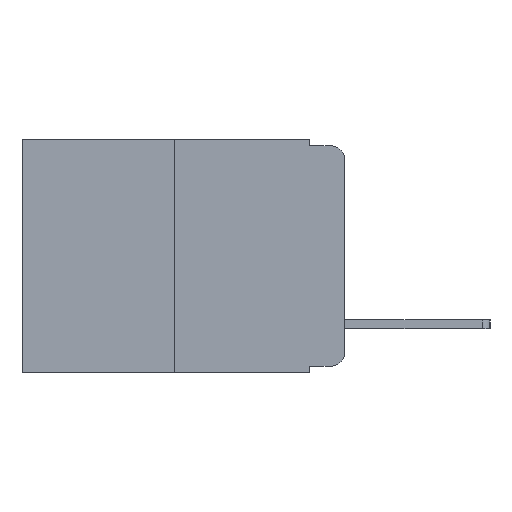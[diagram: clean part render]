
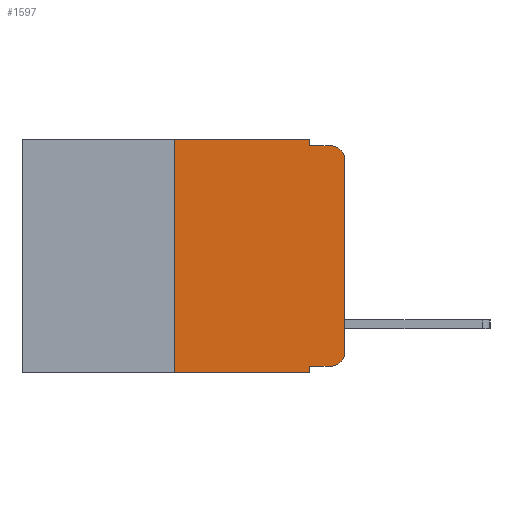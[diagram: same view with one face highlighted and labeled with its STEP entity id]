
A CAD part, left-side view. The second image highlights one B-rep face of the part: STEP entity #1597.
In plain terms, the highlighted planar face has unit normal (-1, 0, 0).
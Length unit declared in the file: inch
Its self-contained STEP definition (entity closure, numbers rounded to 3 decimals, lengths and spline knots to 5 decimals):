
#398 = CARTESIAN_POINT ( 'NONE',  ( 0., 0.25, 0. ) ) ;
#484 = VERTEX_POINT ( 'NONE', #3550 ) ;
#619 = VECTOR ( 'NONE', #3246, 39.37008 ) ;
#721 = ORIENTED_EDGE ( 'NONE', *, *, #3260, .T. ) ;
#739 = CARTESIAN_POINT ( 'NONE',  ( 0., 0.051, -0.01 ) ) ;
#903 = DIRECTION ( 'NONE',  ( 0., 0., -1. ) ) ;
#1189 = VERTEX_POINT ( 'NONE', #8719 ) ;
#1519 = ORIENTED_EDGE ( 'NONE', *, *, #9835, .F. ) ;
#1597 = ADVANCED_FACE ( 'NONE', ( #6270 ), #5409, .F. ) ;
#1646 = DIRECTION ( 'NONE',  ( -1., 0., 0. ) ) ;
#1686 = VECTOR ( 'NONE', #3422, 39.37008 ) ;
#1715 = EDGE_CURVE ( 'NONE', #10775, #1189, #11585, .T. ) ;
#1769 = CARTESIAN_POINT ( 'NONE',  ( 0., 0.02, -0.03 ) ) ;
#1827 = LINE ( 'NONE', #9334, #11790 ) ;
#1900 = CARTESIAN_POINT ( 'NONE',  ( 0., 0., -0.03 ) ) ;
#1905 = EDGE_CURVE ( 'NONE', #6234, #3204, #8114, .T. ) ;
#2061 = LINE ( 'NONE', #12722, #1686 ) ;
#2148 = CARTESIAN_POINT ( 'NONE',  ( 0., 0., 0. ) ) ;
#2688 = LINE ( 'NONE', #739, #12194 ) ;
#2775 = CARTESIAN_POINT ( 'NONE',  ( 0., 0.473, 0. ) ) ;
#2866 = DIRECTION ( 'NONE',  ( 0., 0., 1. ) ) ;
#2919 = CARTESIAN_POINT ( 'NONE',  ( 0., 0.25, 0. ) ) ;
#3045 = CARTESIAN_POINT ( 'NONE',  ( 0., 0.02, -0.333 ) ) ;
#3204 = VERTEX_POINT ( 'NONE', #9785 ) ;
#3246 = DIRECTION ( 'NONE',  ( 0., 0., 1. ) ) ;
#3260 = EDGE_CURVE ( 'NONE', #6850, #10775, #11193, .T. ) ;
#3422 = DIRECTION ( 'NONE',  ( 0., 0., -1. ) ) ;
#3436 = VECTOR ( 'NONE', #7739, 39.37008 ) ;
#3550 = CARTESIAN_POINT ( 'NONE',  ( 0., 0.051, -0.343 ) ) ;
#3652 = VECTOR ( 'NONE', #2866, 39.37008 ) ;
#3736 = DIRECTION ( 'NONE',  ( 0., 0., -1. ) ) ;
#4251 = CARTESIAN_POINT ( 'NONE',  ( 0., 0.473, 0. ) ) ;
#4259 = VECTOR ( 'NONE', #12561, 39.37008 ) ;
#4272 = CARTESIAN_POINT ( 'NONE',  ( 0., 0.473, -0.343 ) ) ;
#4523 = EDGE_LOOP ( 'NONE', ( #721, #9662, #6230, #8957, #7937, #1519, #6076, #11260, #7796, #5656 ) ) ;
#5246 = DIRECTION ( 'NONE',  ( 0., -1., 0. ) ) ;
#5387 = DIRECTION ( 'NONE',  ( 0., 0., -1. ) ) ;
#5396 = VECTOR ( 'NONE', #5246, 39.37008 ) ;
#5409 = PLANE ( 'NONE',  #8946 ) ;
#5447 = DIRECTION ( 'NONE',  ( 1., 0., 0. ) ) ;
#5606 = CARTESIAN_POINT ( 'NONE',  ( 0., 0.051, -0.01 ) ) ;
#5656 = ORIENTED_EDGE ( 'NONE', *, *, #7387, .T. ) ;
#5916 = AXIS2_PLACEMENT_3D ( 'NONE', #12597, #7128, #903 ) ;
#6045 = LINE ( 'NONE', #11411, #3436 ) ;
#6076 = ORIENTED_EDGE ( 'NONE', *, *, #12364, .T. ) ;
#6230 = ORIENTED_EDGE ( 'NONE', *, *, #12300, .F. ) ;
#6234 = VERTEX_POINT ( 'NONE', #398 ) ;
#6270 = FACE_OUTER_BOUND ( 'NONE', #4523, .T. ) ;
#6274 = VERTEX_POINT ( 'NONE', #7692 ) ;
#6453 = CARTESIAN_POINT ( 'NONE',  ( 0., 0., -0.313 ) ) ;
#6739 = LINE ( 'NONE', #4272, #4259 ) ;
#6822 = DIRECTION ( 'NONE',  ( 0., 0., -1. ) ) ;
#6850 = VERTEX_POINT ( 'NONE', #6453 ) ;
#7128 = DIRECTION ( 'NONE',  ( -1., 0., 0. ) ) ;
#7221 = CIRCLE ( 'NONE', #5916, 0.02 ) ;
#7387 = EDGE_CURVE ( 'NONE', #10761, #6850, #7221, .T. ) ;
#7692 = CARTESIAN_POINT ( 'NONE',  ( 0., 0.25, -0.343 ) ) ;
#7739 = DIRECTION ( 'NONE',  ( 0., -1., 0. ) ) ;
#7796 = ORIENTED_EDGE ( 'NONE', *, *, #7978, .T. ) ;
#7905 = DIRECTION ( 'NONE',  ( 0., -1., 0. ) ) ;
#7937 = ORIENTED_EDGE ( 'NONE', *, *, #1905, .F. ) ;
#7978 = EDGE_CURVE ( 'NONE', #8637, #10761, #6045, .T. ) ;
#8114 = LINE ( 'NONE', #4251, #5396 ) ;
#8637 = VERTEX_POINT ( 'NONE', #9374 ) ;
#8651 = LINE ( 'NONE', #2919, #3652 ) ;
#8719 = CARTESIAN_POINT ( 'NONE',  ( 0., 0.02, -0.01 ) ) ;
#8946 = AXIS2_PLACEMENT_3D ( 'NONE', #2775, #5447, #5387 ) ;
#8957 = ORIENTED_EDGE ( 'NONE', *, *, #11095, .F. ) ;
#9218 = EDGE_CURVE ( 'NONE', #8637, #484, #2061, .T. ) ;
#9334 = CARTESIAN_POINT ( 'NONE',  ( 0., 0.051, 0. ) ) ;
#9374 = CARTESIAN_POINT ( 'NONE',  ( 0., 0.051, -0.333 ) ) ;
#9662 = ORIENTED_EDGE ( 'NONE', *, *, #1715, .T. ) ;
#9785 = CARTESIAN_POINT ( 'NONE',  ( 0., 0.051, 0. ) ) ;
#9835 = EDGE_CURVE ( 'NONE', #6274, #6234, #8651, .T. ) ;
#9943 = AXIS2_PLACEMENT_3D ( 'NONE', #1769, #1646, #6822 ) ;
#10761 = VERTEX_POINT ( 'NONE', #3045 ) ;
#10775 = VERTEX_POINT ( 'NONE', #1900 ) ;
#11095 = EDGE_CURVE ( 'NONE', #3204, #11879, #1827, .T. ) ;
#11193 = LINE ( 'NONE', #2148, #619 ) ;
#11260 = ORIENTED_EDGE ( 'NONE', *, *, #9218, .F. ) ;
#11411 = CARTESIAN_POINT ( 'NONE',  ( 0., 0.051, -0.333 ) ) ;
#11585 = CIRCLE ( 'NONE', #9943, 0.02 ) ;
#11790 = VECTOR ( 'NONE', #3736, 39.37008 ) ;
#11879 = VERTEX_POINT ( 'NONE', #5606 ) ;
#12194 = VECTOR ( 'NONE', #7905, 39.37008 ) ;
#12300 = EDGE_CURVE ( 'NONE', #11879, #1189, #2688, .T. ) ;
#12364 = EDGE_CURVE ( 'NONE', #6274, #484, #6739, .T. ) ;
#12561 = DIRECTION ( 'NONE',  ( 0., -1., 0. ) ) ;
#12597 = CARTESIAN_POINT ( 'NONE',  ( 0., 0.02, -0.313 ) ) ;
#12722 = CARTESIAN_POINT ( 'NONE',  ( 0., 0.051, 0. ) ) ;
